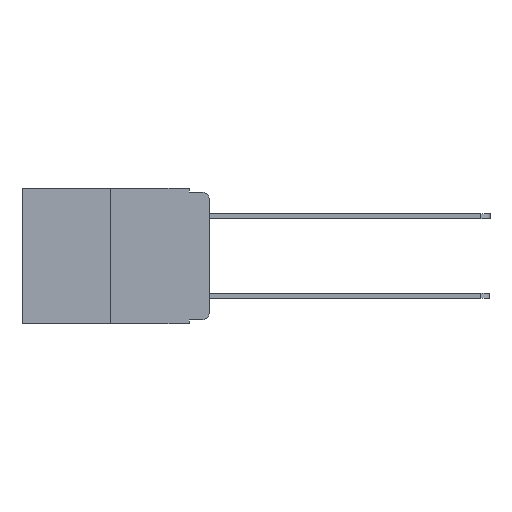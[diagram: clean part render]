
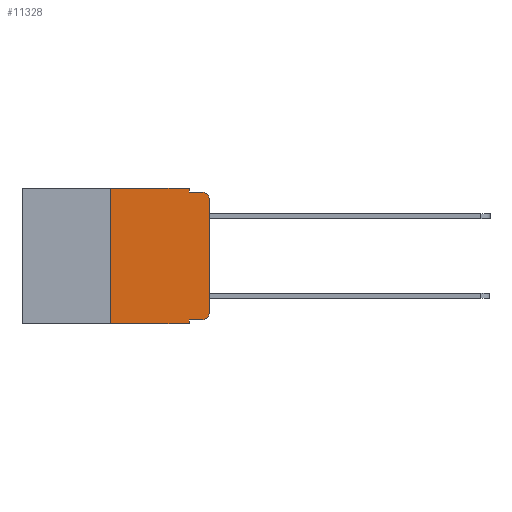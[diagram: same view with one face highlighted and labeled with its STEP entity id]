
A CAD part, left-side view. The second image highlights one B-rep face of the part: STEP entity #11328.
In plain terms, the highlighted planar face has unit normal (-1, 0, 0).
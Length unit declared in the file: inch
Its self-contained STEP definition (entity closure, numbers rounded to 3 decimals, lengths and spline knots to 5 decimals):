
#653 = CARTESIAN_POINT ( 'NONE',  ( 0., 0.02, -0.03 ) ) ;
#844 = VERTEX_POINT ( 'NONE', #1902 ) ;
#1429 = LINE ( 'NONE', #3528, #8258 ) ;
#1729 = DIRECTION ( 'NONE',  ( 0., 0., -1. ) ) ;
#1789 = VERTEX_POINT ( 'NONE', #7491 ) ;
#1902 = CARTESIAN_POINT ( 'NONE',  ( 0., 0.25, -0.343 ) ) ;
#2049 = LINE ( 'NONE', #10496, #6749 ) ;
#2103 = VERTEX_POINT ( 'NONE', #2924 ) ;
#2195 = VERTEX_POINT ( 'NONE', #2254 ) ;
#2254 = CARTESIAN_POINT ( 'NONE',  ( 0., 0., -0.03 ) ) ;
#2318 = DIRECTION ( 'NONE',  ( 0., -1., 0. ) ) ;
#2323 = VECTOR ( 'NONE', #10983, 39.37008 ) ;
#2398 = ORIENTED_EDGE ( 'NONE', *, *, #5243, .T. ) ;
#2496 = ORIENTED_EDGE ( 'NONE', *, *, #10902, .T. ) ;
#2585 = CARTESIAN_POINT ( 'NONE',  ( 0., 0.473, -0.343 ) ) ;
#2599 = CARTESIAN_POINT ( 'NONE',  ( 0., 0.051, -0.01 ) ) ;
#2708 = VERTEX_POINT ( 'NONE', #5627 ) ;
#2751 = ORIENTED_EDGE ( 'NONE', *, *, #9859, .T. ) ;
#2775 = CARTESIAN_POINT ( 'NONE',  ( 0., 0.25, 0. ) ) ;
#2852 = EDGE_LOOP ( 'NONE', ( #2496, #2751, #3783, #4470, #5144, #3857, #4902, #6078, #2398, #2881 ) ) ;
#2881 = ORIENTED_EDGE ( 'NONE', *, *, #4636, .T. ) ;
#2924 = CARTESIAN_POINT ( 'NONE',  ( 0., 0.051, -0.333 ) ) ;
#3012 = LINE ( 'NONE', #4569, #9770 ) ;
#3063 = CARTESIAN_POINT ( 'NONE',  ( 0., 0.473, 0. ) ) ;
#3278 = DIRECTION ( 'NONE',  ( 0., 0., 1. ) ) ;
#3528 = CARTESIAN_POINT ( 'NONE',  ( 0., 0., 0. ) ) ;
#3567 = AXIS2_PLACEMENT_3D ( 'NONE', #653, #7335, #1729 ) ;
#3701 = CIRCLE ( 'NONE', #3567, 0.02 ) ;
#3721 = LINE ( 'NONE', #9498, #5839 ) ;
#3749 = VERTEX_POINT ( 'NONE', #6541 ) ;
#3783 = ORIENTED_EDGE ( 'NONE', *, *, #8786, .F. ) ;
#3857 = ORIENTED_EDGE ( 'NONE', *, *, #7040, .F. ) ;
#4440 = VERTEX_POINT ( 'NONE', #5840 ) ;
#4470 = ORIENTED_EDGE ( 'NONE', *, *, #8202, .F. ) ;
#4499 = DIRECTION ( 'NONE',  ( 0., -1., 0. ) ) ;
#4569 = CARTESIAN_POINT ( 'NONE',  ( 0., 0.051, 0. ) ) ;
#4636 = EDGE_CURVE ( 'NONE', #3749, #5045, #9435, .T. ) ;
#4863 = LINE ( 'NONE', #9421, #2323 ) ;
#4902 = ORIENTED_EDGE ( 'NONE', *, *, #7782, .T. ) ;
#5045 = VERTEX_POINT ( 'NONE', #11056 ) ;
#5091 = VERTEX_POINT ( 'NONE', #2775 ) ;
#5144 = ORIENTED_EDGE ( 'NONE', *, *, #9601, .F. ) ;
#5243 = EDGE_CURVE ( 'NONE', #2103, #3749, #2049, .T. ) ;
#5357 = DIRECTION ( 'NONE',  ( 0., 0., 1. ) ) ;
#5585 = LINE ( 'NONE', #8624, #9878 ) ;
#5627 = CARTESIAN_POINT ( 'NONE',  ( 0., 0.02, -0.01 ) ) ;
#5826 = DIRECTION ( 'NONE',  ( 1., 0., 0. ) ) ;
#5839 = VECTOR ( 'NONE', #6077, 39.37008 ) ;
#5840 = CARTESIAN_POINT ( 'NONE',  ( 0., 0.051, 0. ) ) ;
#6077 = DIRECTION ( 'NONE',  ( 0., 0., -1. ) ) ;
#6078 = ORIENTED_EDGE ( 'NONE', *, *, #6444, .F. ) ;
#6245 = LINE ( 'NONE', #9509, #10444 ) ;
#6444 = EDGE_CURVE ( 'NONE', #2103, #1789, #3012, .T. ) ;
#6541 = CARTESIAN_POINT ( 'NONE',  ( 0., 0.02, -0.333 ) ) ;
#6749 = VECTOR ( 'NONE', #10789, 39.37008 ) ;
#7035 = FACE_OUTER_BOUND ( 'NONE', #2852, .T. ) ;
#7040 = EDGE_CURVE ( 'NONE', #844, #5091, #5585, .T. ) ;
#7238 = VERTEX_POINT ( 'NONE', #2599 ) ;
#7335 = DIRECTION ( 'NONE',  ( -1., 0., 0. ) ) ;
#7491 = CARTESIAN_POINT ( 'NONE',  ( 0., 0.051, -0.343 ) ) ;
#7782 = EDGE_CURVE ( 'NONE', #844, #1789, #9860, .T. ) ;
#8202 = EDGE_CURVE ( 'NONE', #4440, #7238, #3721, .T. ) ;
#8258 = VECTOR ( 'NONE', #5357, 39.37008 ) ;
#8407 = DIRECTION ( 'NONE',  ( 0., 0., -1. ) ) ;
#8624 = CARTESIAN_POINT ( 'NONE',  ( 0., 0.25, 0. ) ) ;
#8786 = EDGE_CURVE ( 'NONE', #7238, #2708, #4863, .T. ) ;
#8820 = DIRECTION ( 'NONE',  ( 0., 0., -1. ) ) ;
#8827 = DIRECTION ( 'NONE',  ( -1., 0., 0. ) ) ;
#8848 = CARTESIAN_POINT ( 'NONE',  ( 0., 0.02, -0.313 ) ) ;
#8864 = AXIS2_PLACEMENT_3D ( 'NONE', #3063, #5826, #11587 ) ;
#9368 = VECTOR ( 'NONE', #4499, 39.37008 ) ;
#9421 = CARTESIAN_POINT ( 'NONE',  ( 0., 0.051, -0.01 ) ) ;
#9435 = CIRCLE ( 'NONE', #11175, 0.02 ) ;
#9498 = CARTESIAN_POINT ( 'NONE',  ( 0., 0.051, 0. ) ) ;
#9509 = CARTESIAN_POINT ( 'NONE',  ( 0., 0.473, 0. ) ) ;
#9601 = EDGE_CURVE ( 'NONE', #5091, #4440, #6245, .T. ) ;
#9770 = VECTOR ( 'NONE', #8407, 39.37008 ) ;
#9859 = EDGE_CURVE ( 'NONE', #2195, #2708, #3701, .T. ) ;
#9860 = LINE ( 'NONE', #2585, #9368 ) ;
#9878 = VECTOR ( 'NONE', #3278, 39.37008 ) ;
#10444 = VECTOR ( 'NONE', #2318, 39.37008 ) ;
#10496 = CARTESIAN_POINT ( 'NONE',  ( 0., 0.051, -0.333 ) ) ;
#10789 = DIRECTION ( 'NONE',  ( 0., -1., 0. ) ) ;
#10851 = PLANE ( 'NONE',  #8864 ) ;
#10902 = EDGE_CURVE ( 'NONE', #5045, #2195, #1429, .T. ) ;
#10983 = DIRECTION ( 'NONE',  ( 0., -1., 0. ) ) ;
#11056 = CARTESIAN_POINT ( 'NONE',  ( 0., 0., -0.313 ) ) ;
#11175 = AXIS2_PLACEMENT_3D ( 'NONE', #8848, #8827, #8820 ) ;
#11328 = ADVANCED_FACE ( 'NONE', ( #7035 ), #10851, .F. ) ;
#11587 = DIRECTION ( 'NONE',  ( 0., 0., -1. ) ) ;
